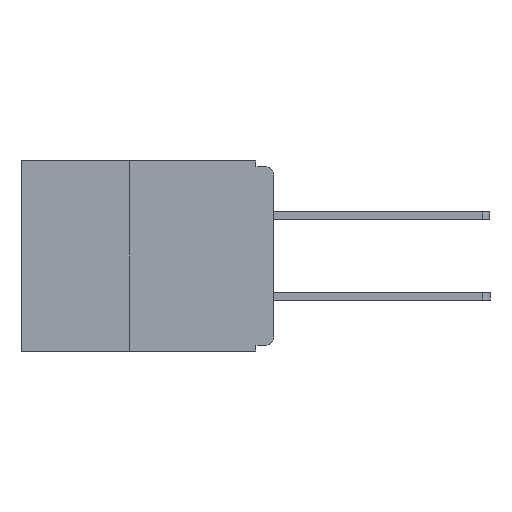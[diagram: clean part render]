
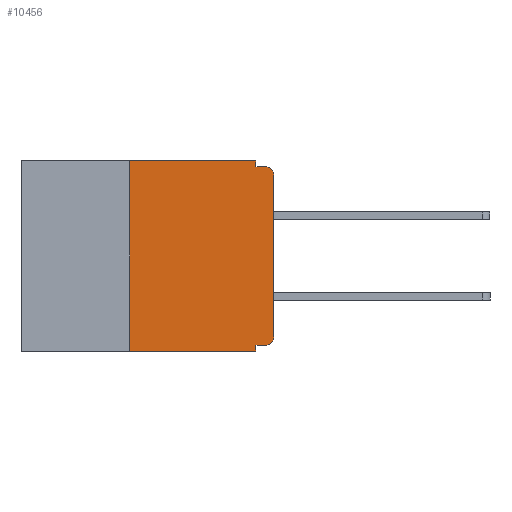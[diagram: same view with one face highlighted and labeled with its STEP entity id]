
A CAD part, left-side view. The second image highlights one B-rep face of the part: STEP entity #10456.
In plain terms, the highlighted planar face has unit normal (-1, 0, 0).
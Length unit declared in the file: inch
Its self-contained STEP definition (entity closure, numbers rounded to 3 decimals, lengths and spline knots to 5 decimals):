
#152 = VERTEX_POINT ( 'NONE', #18697 ) ;
#176 = DIRECTION ( 'NONE',  ( 0., 0., -1. ) ) ;
#277 = CARTESIAN_POINT ( 'NONE',  ( 0., 0.031, 0. ) ) ;
#640 = VERTEX_POINT ( 'NONE', #4020 ) ;
#740 = CARTESIAN_POINT ( 'NONE',  ( 0., 0.25, -0.33 ) ) ;
#1791 = DIRECTION ( 'NONE',  ( 0., 0., -1. ) ) ;
#1814 = DIRECTION ( 'NONE',  ( 1., 0., 0. ) ) ;
#1858 = CARTESIAN_POINT ( 'NONE',  ( 0., 0.437, 0. ) ) ;
#1988 = PLANE ( 'NONE',  #9297 ) ;
#2239 = LINE ( 'NONE', #17716, #6156 ) ;
#2313 = VECTOR ( 'NONE', #15563, 39.37008 ) ;
#2838 = DIRECTION ( 'NONE',  ( 0., -1., 0. ) ) ;
#2988 = CARTESIAN_POINT ( 'NONE',  ( 0., 0.437, 0. ) ) ;
#4020 = CARTESIAN_POINT ( 'NONE',  ( 0., 0.25, -0.33 ) ) ;
#4049 = ORIENTED_EDGE ( 'NONE', *, *, #6194, .T. ) ;
#4214 = VERTEX_POINT ( 'NONE', #13516 ) ;
#4220 = VERTEX_POINT ( 'NONE', #13191 ) ;
#4341 = ORIENTED_EDGE ( 'NONE', *, *, #19726, .T. ) ;
#4457 = ORIENTED_EDGE ( 'NONE', *, *, #18635, .F. ) ;
#4535 = LINE ( 'NONE', #17910, #17144 ) ;
#4724 = VECTOR ( 'NONE', #17149, 39.37008 ) ;
#4815 = ORIENTED_EDGE ( 'NONE', *, *, #16477, .F. ) ;
#5096 = ORIENTED_EDGE ( 'NONE', *, *, #11460, .F. ) ;
#5252 = LINE ( 'NONE', #18724, #4724 ) ;
#5254 = VECTOR ( 'NONE', #15754, 39.37008 ) ;
#5285 = LINE ( 'NONE', #10822, #6828 ) ;
#5391 = ORIENTED_EDGE ( 'NONE', *, *, #14329, .F. ) ;
#5711 = ORIENTED_EDGE ( 'NONE', *, *, #12097, .T. ) ;
#5877 = ORIENTED_EDGE ( 'NONE', *, *, #8795, .F. ) ;
#6072 = CARTESIAN_POINT ( 'NONE',  ( 0., 0., -0.025 ) ) ;
#6156 = VECTOR ( 'NONE', #17595, 39.37008 ) ;
#6194 = EDGE_CURVE ( 'NONE', #152, #8978, #2239, .T. ) ;
#6270 = CARTESIAN_POINT ( 'NONE',  ( 0., 0.25, 0. ) ) ;
#6700 = LINE ( 'NONE', #19799, #14964 ) ;
#6828 = VECTOR ( 'NONE', #10221, 39.37008 ) ;
#7434 = ORIENTED_EDGE ( 'NONE', *, *, #11024, .F. ) ;
#7767 = LINE ( 'NONE', #2988, #11107 ) ;
#7940 = EDGE_LOOP ( 'NONE', ( #4049, #4341, #4457, #4815, #5096, #5391, #5711, #5877, #7434, #7969 ) ) ;
#7969 = ORIENTED_EDGE ( 'NONE', *, *, #16631, .T. ) ;
#8318 = CIRCLE ( 'NONE', #12469, 0.015 ) ;
#8758 = VERTEX_POINT ( 'NONE', #11026 ) ;
#8795 = EDGE_CURVE ( 'NONE', #4220, #8758, #5285, .T. ) ;
#8817 = CARTESIAN_POINT ( 'NONE',  ( 0., 0.015, -0.025 ) ) ;
#8978 = VERTEX_POINT ( 'NONE', #6072 ) ;
#8980 = CARTESIAN_POINT ( 'NONE',  ( 0., 0.015, -0.305 ) ) ;
#9297 = AXIS2_PLACEMENT_3D ( 'NONE', #1858, #1814, #1791 ) ;
#9784 = DIRECTION ( 'NONE',  ( 0., -1., 0. ) ) ;
#10065 = VERTEX_POINT ( 'NONE', #6270 ) ;
#10221 = DIRECTION ( 'NONE',  ( 0., 0., -1. ) ) ;
#10455 = DIRECTION ( 'NONE',  ( 0., 0., -1. ) ) ;
#10456 = ADVANCED_FACE ( 'NONE', ( #14277 ), #1988, .F. ) ;
#10580 = VERTEX_POINT ( 'NONE', #277 ) ;
#10621 = DIRECTION ( 'NONE',  ( 0., 0., -1. ) ) ;
#10822 = CARTESIAN_POINT ( 'NONE',  ( 0., 0.031, -0.33 ) ) ;
#11024 = EDGE_CURVE ( 'NONE', #4214, #4220, #20116, .T. ) ;
#11026 = CARTESIAN_POINT ( 'NONE',  ( 0., 0.031, -0.33 ) ) ;
#11107 = VECTOR ( 'NONE', #2838, 39.37008 ) ;
#11460 = EDGE_CURVE ( 'NONE', #10065, #10580, #7767, .T. ) ;
#12097 = EDGE_CURVE ( 'NONE', #640, #8758, #4535, .T. ) ;
#12254 = CARTESIAN_POINT ( 'NONE',  ( 0., 0.031, -0.01 ) ) ;
#12469 = AXIS2_PLACEMENT_3D ( 'NONE', #8817, #20037, #10455 ) ;
#13191 = CARTESIAN_POINT ( 'NONE',  ( 0., 0.031, -0.32 ) ) ;
#13419 = CIRCLE ( 'NONE', #16259, 0.015 ) ;
#13516 = CARTESIAN_POINT ( 'NONE',  ( 0., 0.015, -0.32 ) ) ;
#13666 = VERTEX_POINT ( 'NONE', #16963 ) ;
#14066 = LINE ( 'NONE', #740, #5254 ) ;
#14277 = FACE_OUTER_BOUND ( 'NONE', #7940, .T. ) ;
#14329 = EDGE_CURVE ( 'NONE', #640, #10065, #14066, .T. ) ;
#14964 = VECTOR ( 'NONE', #176, 39.37008 ) ;
#15059 = CARTESIAN_POINT ( 'NONE',  ( 0., 0., -0.32 ) ) ;
#15563 = DIRECTION ( 'NONE',  ( 0., 1., 0. ) ) ;
#15754 = DIRECTION ( 'NONE',  ( 0., 0., 1. ) ) ;
#16259 = AXIS2_PLACEMENT_3D ( 'NONE', #8980, #20195, #10621 ) ;
#16477 = EDGE_CURVE ( 'NONE', #10580, #19787, #6700, .T. ) ;
#16631 = EDGE_CURVE ( 'NONE', #4214, #152, #13419, .T. ) ;
#16963 = CARTESIAN_POINT ( 'NONE',  ( 0., 0.015, -0.01 ) ) ;
#17144 = VECTOR ( 'NONE', #9784, 39.37008 ) ;
#17149 = DIRECTION ( 'NONE',  ( 0., -1., 0. ) ) ;
#17595 = DIRECTION ( 'NONE',  ( 0., 0., 1. ) ) ;
#17716 = CARTESIAN_POINT ( 'NONE',  ( 0., 0., 0. ) ) ;
#17910 = CARTESIAN_POINT ( 'NONE',  ( 0., 0.437, -0.33 ) ) ;
#18635 = EDGE_CURVE ( 'NONE', #19787, #13666, #5252, .T. ) ;
#18697 = CARTESIAN_POINT ( 'NONE',  ( 0., 0., -0.305 ) ) ;
#18724 = CARTESIAN_POINT ( 'NONE',  ( 0., 0., -0.01 ) ) ;
#19726 = EDGE_CURVE ( 'NONE', #8978, #13666, #8318, .T. ) ;
#19787 = VERTEX_POINT ( 'NONE', #12254 ) ;
#19799 = CARTESIAN_POINT ( 'NONE',  ( 0., 0.031, 0. ) ) ;
#20037 = DIRECTION ( 'NONE',  ( -1., 0., 0. ) ) ;
#20116 = LINE ( 'NONE', #15059, #2313 ) ;
#20195 = DIRECTION ( 'NONE',  ( -1., 0., 0. ) ) ;
